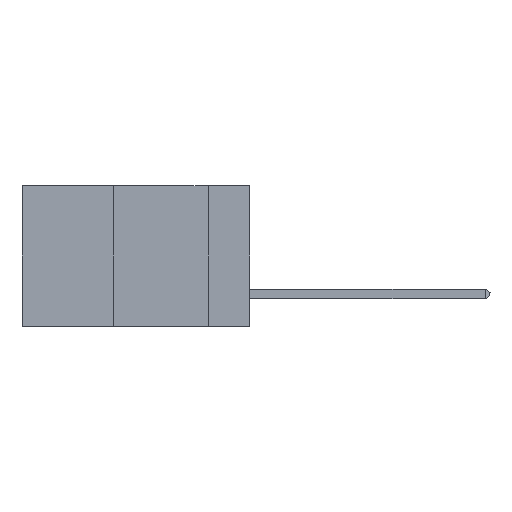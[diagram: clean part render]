
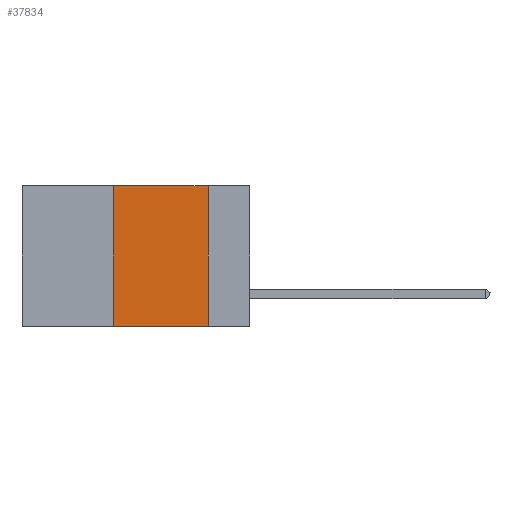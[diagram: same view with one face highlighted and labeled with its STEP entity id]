
A CAD part, left-side view. The second image highlights one B-rep face of the part: STEP entity #37834.
In plain terms, the highlighted planar face has unit normal (-1, 0, 0).
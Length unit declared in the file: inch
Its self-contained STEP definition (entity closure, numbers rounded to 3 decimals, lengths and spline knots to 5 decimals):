
#282 = VECTOR ( 'NONE', #40199, 39.37008 ) ;
#991 = VECTOR ( 'NONE', #38680, 39.37008 ) ;
#2219 = EDGE_LOOP ( 'NONE', ( #14964, #2999, #19727, #15481 ) ) ;
#2999 = ORIENTED_EDGE ( 'NONE', *, *, #18523, .F. ) ;
#4299 = CARTESIAN_POINT ( 'NONE',  ( 0., 0.11, 0. ) ) ;
#5071 = LINE ( 'NONE', #12151, #40698 ) ;
#5669 = DIRECTION ( 'NONE',  ( 0., 0., -1. ) ) ;
#6677 = VERTEX_POINT ( 'NONE', #4299 ) ;
#9188 = PLANE ( 'NONE',  #25606 ) ;
#9254 = LINE ( 'NONE', #26723, #282 ) ;
#12151 = CARTESIAN_POINT ( 'NONE',  ( 0., 0.11, 0. ) ) ;
#12263 = VECTOR ( 'NONE', #28443, 39.37008 ) ;
#12555 = LINE ( 'NONE', #31815, #991 ) ;
#14385 = LINE ( 'NONE', #15317, #12263 ) ;
#14964 = ORIENTED_EDGE ( 'NONE', *, *, #27598, .F. ) ;
#15317 = CARTESIAN_POINT ( 'NONE',  ( 0., 0.36, 0. ) ) ;
#15481 = ORIENTED_EDGE ( 'NONE', *, *, #17126, .T. ) ;
#15960 = CARTESIAN_POINT ( 'NONE',  ( 0., 0.6, 0. ) ) ;
#17126 = EDGE_CURVE ( 'NONE', #24985, #41300, #12555, .T. ) ;
#18523 = EDGE_CURVE ( 'NONE', #25377, #6677, #9254, .T. ) ;
#19727 = ORIENTED_EDGE ( 'NONE', *, *, #40497, .F. ) ;
#24985 = VERTEX_POINT ( 'NONE', #28452 ) ;
#25377 = VERTEX_POINT ( 'NONE', #36748 ) ;
#25606 = AXIS2_PLACEMENT_3D ( 'NONE', #15960, #32612, #32327 ) ;
#26723 = CARTESIAN_POINT ( 'NONE',  ( 0., 0.6, 0. ) ) ;
#27597 = FACE_OUTER_BOUND ( 'NONE', #2219, .T. ) ;
#27598 = EDGE_CURVE ( 'NONE', #6677, #41300, #5071, .T. ) ;
#28443 = DIRECTION ( 'NONE',  ( 0., 0., 1. ) ) ;
#28452 = CARTESIAN_POINT ( 'NONE',  ( 0., 0.36, -0.37 ) ) ;
#31815 = CARTESIAN_POINT ( 'NONE',  ( 0., 0.6, -0.37 ) ) ;
#32327 = DIRECTION ( 'NONE',  ( 0., 0., -1. ) ) ;
#32612 = DIRECTION ( 'NONE',  ( 1., 0., 0. ) ) ;
#36402 = CARTESIAN_POINT ( 'NONE',  ( 0., 0.11, -0.37 ) ) ;
#36748 = CARTESIAN_POINT ( 'NONE',  ( 0., 0.36, 0. ) ) ;
#37834 = ADVANCED_FACE ( 'NONE', ( #27597 ), #9188, .F. ) ;
#38680 = DIRECTION ( 'NONE',  ( 0., -1., 0. ) ) ;
#40199 = DIRECTION ( 'NONE',  ( 0., -1., 0. ) ) ;
#40497 = EDGE_CURVE ( 'NONE', #24985, #25377, #14385, .T. ) ;
#40698 = VECTOR ( 'NONE', #5669, 39.37008 ) ;
#41300 = VERTEX_POINT ( 'NONE', #36402 ) ;
